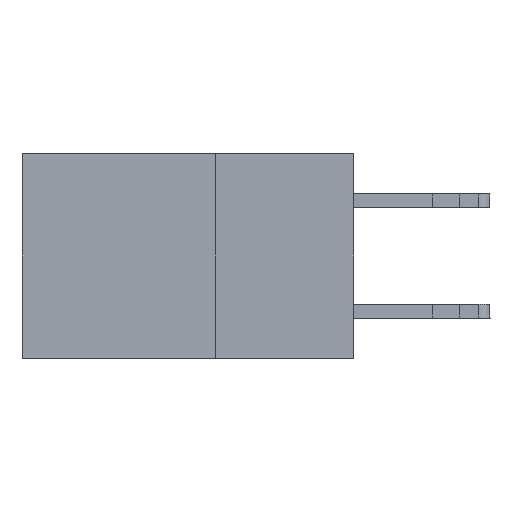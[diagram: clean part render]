
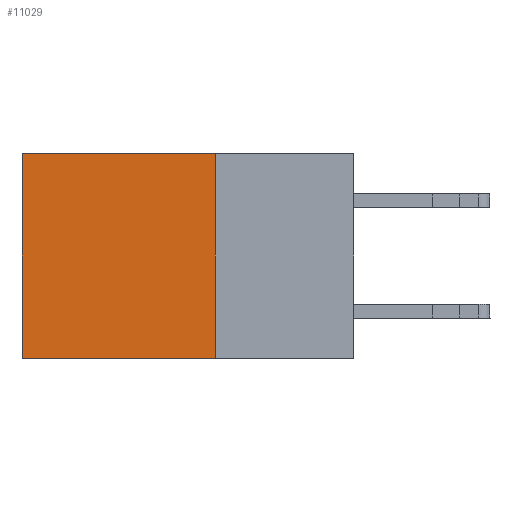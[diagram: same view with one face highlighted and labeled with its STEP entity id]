
A CAD part, left-side view. The second image highlights one B-rep face of the part: STEP entity #11029.
In plain terms, the highlighted planar face has unit normal (-1, 0, 0).
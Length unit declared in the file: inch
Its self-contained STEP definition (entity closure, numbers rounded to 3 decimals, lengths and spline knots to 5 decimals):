
#1691 = VECTOR ( 'NONE', #14306, 39.37008 ) ;
#2232 = VERTEX_POINT ( 'NONE', #8809 ) ;
#2710 = LINE ( 'NONE', #2810, #8290 ) ;
#2804 = CARTESIAN_POINT ( 'NONE',  ( 0.2875, 0.25, 0. ) ) ;
#2810 = CARTESIAN_POINT ( 'NONE',  ( 0.2875, 0.6, 0. ) ) ;
#2954 = LINE ( 'NONE', #15608, #19231 ) ;
#4269 = CARTESIAN_POINT ( 'NONE',  ( 0.2875, 0.25, 0. ) ) ;
#4902 = ORIENTED_EDGE ( 'NONE', *, *, #13738, .F. ) ;
#6185 = DIRECTION ( 'NONE',  ( 0., 1., 0. ) ) ;
#6574 = EDGE_CURVE ( 'NONE', #14226, #2232, #7773, .T. ) ;
#6772 = EDGE_LOOP ( 'NONE', ( #8675, #13489, #4902, #6874 ) ) ;
#6874 = ORIENTED_EDGE ( 'NONE', *, *, #14106, .T. ) ;
#7773 = LINE ( 'NONE', #16066, #1691 ) ;
#8290 = VECTOR ( 'NONE', #10782, 39.37008 ) ;
#8675 = ORIENTED_EDGE ( 'NONE', *, *, #13708, .T. ) ;
#8809 = CARTESIAN_POINT ( 'NONE',  ( 0.2875, 0.6, -0.37 ) ) ;
#10782 = DIRECTION ( 'NONE',  ( 0., 0., -1. ) ) ;
#11029 = ADVANCED_FACE ( 'NONE', ( #11901 ), #14906, .F. ) ;
#11901 = FACE_OUTER_BOUND ( 'NONE', #6772, .T. ) ;
#12007 = CARTESIAN_POINT ( 'NONE',  ( 0.2875, 0.25, 0. ) ) ;
#12438 = VERTEX_POINT ( 'NONE', #2804 ) ;
#12477 = CARTESIAN_POINT ( 'NONE',  ( 0.2875, 0.6, 0. ) ) ;
#13382 = VERTEX_POINT ( 'NONE', #12477 ) ;
#13489 = ORIENTED_EDGE ( 'NONE', *, *, #6574, .F. ) ;
#13708 = EDGE_CURVE ( 'NONE', #13382, #2232, #2710, .T. ) ;
#13738 = EDGE_CURVE ( 'NONE', #12438, #14226, #20127, .T. ) ;
#14106 = EDGE_CURVE ( 'NONE', #12438, #13382, #2954, .T. ) ;
#14226 = VERTEX_POINT ( 'NONE', #15504 ) ;
#14306 = DIRECTION ( 'NONE',  ( 0., 1., 0. ) ) ;
#14906 = PLANE ( 'NONE',  #19619 ) ;
#15356 = DIRECTION ( 'NONE',  ( 0., 0., -1. ) ) ;
#15504 = CARTESIAN_POINT ( 'NONE',  ( 0.2875, 0.25, -0.37 ) ) ;
#15608 = CARTESIAN_POINT ( 'NONE',  ( 0.2875, 0.25, 0. ) ) ;
#16066 = CARTESIAN_POINT ( 'NONE',  ( 0.2875, 0.25, -0.37 ) ) ;
#17912 = DIRECTION ( 'NONE',  ( 1., 0., 0. ) ) ;
#18216 = DIRECTION ( 'NONE',  ( 0., 0., -1. ) ) ;
#19231 = VECTOR ( 'NONE', #6185, 39.37008 ) ;
#19619 = AXIS2_PLACEMENT_3D ( 'NONE', #12007, #17912, #18216 ) ;
#20127 = LINE ( 'NONE', #4269, #20225 ) ;
#20225 = VECTOR ( 'NONE', #15356, 39.37008 ) ;
